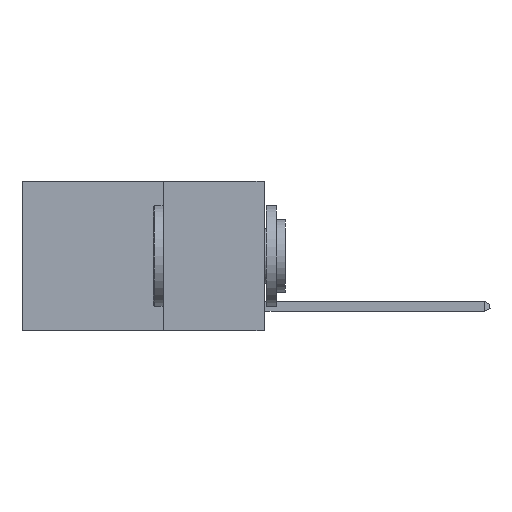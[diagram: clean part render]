
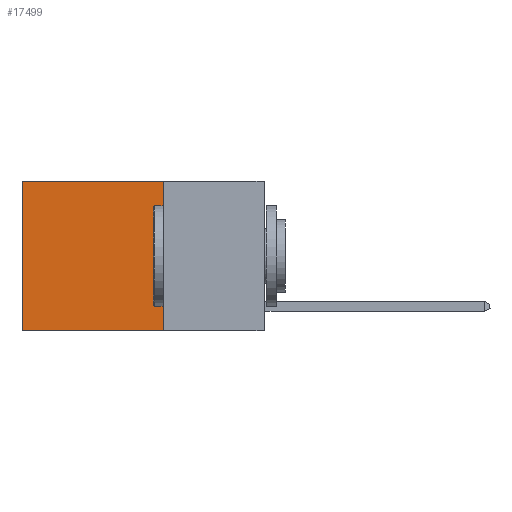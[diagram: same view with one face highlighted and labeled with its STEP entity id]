
A CAD part, left-side view. The second image highlights one B-rep face of the part: STEP entity #17499.
In plain terms, the highlighted planar face has unit normal (-1, 0, 0).
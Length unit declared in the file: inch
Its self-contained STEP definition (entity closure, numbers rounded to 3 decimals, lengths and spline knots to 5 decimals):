
#695 = LINE ( 'NONE', #5444, #2919 ) ;
#933 = EDGE_CURVE ( 'NONE', #17243, #21280, #14303, .T. ) ;
#1557 = ORIENTED_EDGE ( 'NONE', *, *, #7763, .T. ) ;
#1896 = FACE_OUTER_BOUND ( 'NONE', #16125, .T. ) ;
#2911 = CARTESIAN_POINT ( 'NONE',  ( 0.2625, 0.25, 0. ) ) ;
#2919 = VECTOR ( 'NONE', #5345, 39.37008 ) ;
#2985 = CARTESIAN_POINT ( 'NONE',  ( 0.2625, 0.25, 0. ) ) ;
#3714 = AXIS2_PLACEMENT_3D ( 'NONE', #13807, #7052, #18677 ) ;
#4252 = LINE ( 'NONE', #9103, #6674 ) ;
#4847 = VERTEX_POINT ( 'NONE', #2911 ) ;
#5334 = ORIENTED_EDGE ( 'NONE', *, *, #9050, .F. ) ;
#5345 = DIRECTION ( 'NONE',  ( 0., 0., -1. ) ) ;
#5444 = CARTESIAN_POINT ( 'NONE',  ( 0.2625, 0.6, 0. ) ) ;
#5798 = VERTEX_POINT ( 'NONE', #9908 ) ;
#5888 = DIRECTION ( 'NONE',  ( 0., 0., -1. ) ) ;
#6674 = VECTOR ( 'NONE', #5888, 39.37008 ) ;
#7052 = DIRECTION ( 'NONE',  ( 1., 0., 0. ) ) ;
#7763 = EDGE_CURVE ( 'NONE', #5798, #21280, #695, .T. ) ;
#7842 = CARTESIAN_POINT ( 'NONE',  ( 0.2625, 0.25, -0.37 ) ) ;
#9050 = EDGE_CURVE ( 'NONE', #4847, #17243, #4252, .T. ) ;
#9103 = CARTESIAN_POINT ( 'NONE',  ( 0.2625, 0.25, 0. ) ) ;
#9725 = DIRECTION ( 'NONE',  ( 0., 1., 0. ) ) ;
#9908 = CARTESIAN_POINT ( 'NONE',  ( 0.2625, 0.6, 0. ) ) ;
#10100 = ORIENTED_EDGE ( 'NONE', *, *, #933, .F. ) ;
#11317 = EDGE_CURVE ( 'NONE', #4847, #5798, #18126, .T. ) ;
#13807 = CARTESIAN_POINT ( 'NONE',  ( 0.2625, 0.25, 0. ) ) ;
#14303 = LINE ( 'NONE', #17634, #15210 ) ;
#15210 = VECTOR ( 'NONE', #15760, 39.37008 ) ;
#15760 = DIRECTION ( 'NONE',  ( 0., 1., 0. ) ) ;
#16125 = EDGE_LOOP ( 'NONE', ( #1557, #10100, #5334, #19568 ) ) ;
#16792 = PLANE ( 'NONE',  #3714 ) ;
#17243 = VERTEX_POINT ( 'NONE', #7842 ) ;
#17373 = VECTOR ( 'NONE', #9725, 39.37008 ) ;
#17499 = ADVANCED_FACE ( 'NONE', ( #1896 ), #16792, .F. ) ;
#17634 = CARTESIAN_POINT ( 'NONE',  ( 0.2625, 0.25, -0.37 ) ) ;
#18126 = LINE ( 'NONE', #2985, #17373 ) ;
#18677 = DIRECTION ( 'NONE',  ( 0., 0., -1. ) ) ;
#19568 = ORIENTED_EDGE ( 'NONE', *, *, #11317, .T. ) ;
#19925 = CARTESIAN_POINT ( 'NONE',  ( 0.2625, 0.6, -0.37 ) ) ;
#21280 = VERTEX_POINT ( 'NONE', #19925 ) ;
